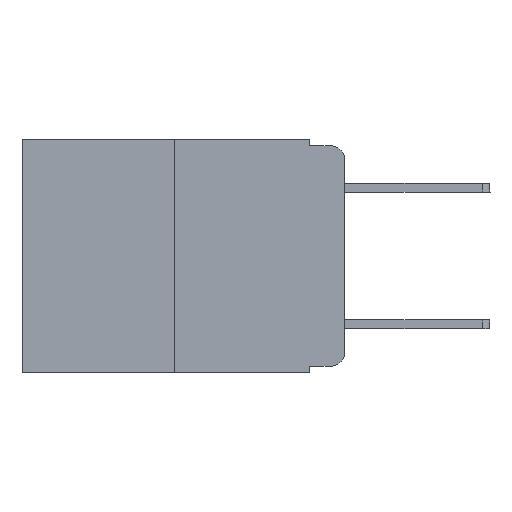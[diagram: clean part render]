
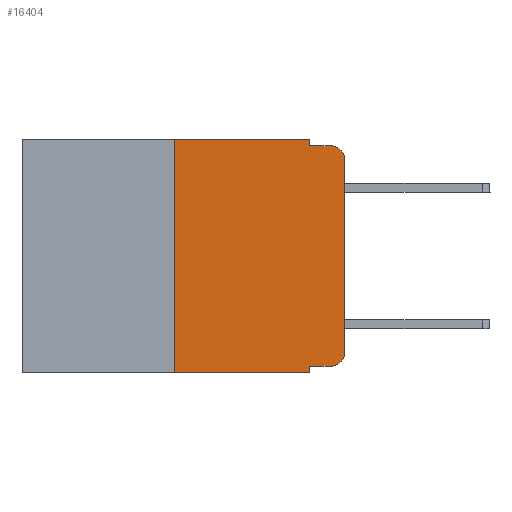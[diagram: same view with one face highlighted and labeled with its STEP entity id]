
A CAD part, left-side view. The second image highlights one B-rep face of the part: STEP entity #16404.
In plain terms, the highlighted planar face has unit normal (-1, 0, 0).
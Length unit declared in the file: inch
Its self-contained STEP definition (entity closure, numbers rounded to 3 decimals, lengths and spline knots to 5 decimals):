
#246 = AXIS2_PLACEMENT_3D ( 'NONE', #10239, #17850, #14669 ) ;
#283 = LINE ( 'NONE', #13062, #1094 ) ;
#313 = VERTEX_POINT ( 'NONE', #12540 ) ;
#344 = CARTESIAN_POINT ( 'NONE',  ( 0., 0.25, 0. ) ) ;
#580 = DIRECTION ( 'NONE',  ( 0., -1., 0. ) ) ;
#756 = VECTOR ( 'NONE', #9069, 39.37008 ) ;
#832 = ORIENTED_EDGE ( 'NONE', *, *, #17489, .T. ) ;
#1014 = CARTESIAN_POINT ( 'NONE',  ( 0., 0., -0.313 ) ) ;
#1094 = VECTOR ( 'NONE', #7331, 39.37008 ) ;
#1311 = ORIENTED_EDGE ( 'NONE', *, *, #4540, .T. ) ;
#1419 = DIRECTION ( 'NONE',  ( -1., 0., 0. ) ) ;
#1747 = CIRCLE ( 'NONE', #246, 0.02 ) ;
#2169 = EDGE_CURVE ( 'NONE', #313, #12812, #13133, .T. ) ;
#2287 = VECTOR ( 'NONE', #17711, 39.37008 ) ;
#2342 = EDGE_CURVE ( 'NONE', #17823, #13980, #2586, .T. ) ;
#2538 = DIRECTION ( 'NONE',  ( 0., 0., -1. ) ) ;
#2543 = DIRECTION ( 'NONE',  ( 0., -1., 0. ) ) ;
#2586 = LINE ( 'NONE', #13967, #7537 ) ;
#2757 = CARTESIAN_POINT ( 'NONE',  ( 0., 0.051, 0. ) ) ;
#2827 = CARTESIAN_POINT ( 'NONE',  ( 0., 0.02, -0.03 ) ) ;
#2892 = VERTEX_POINT ( 'NONE', #8205 ) ;
#3056 = VECTOR ( 'NONE', #3550, 39.37008 ) ;
#3317 = LINE ( 'NONE', #7725, #13115 ) ;
#3349 = LINE ( 'NONE', #17541, #756 ) ;
#3550 = DIRECTION ( 'NONE',  ( 0., -1., 0. ) ) ;
#4470 = EDGE_LOOP ( 'NONE', ( #15710, #832, #5228, #12486, #15642, #16694, #1311, #16005, #11245, #15691 ) ) ;
#4540 = EDGE_CURVE ( 'NONE', #14877, #2892, #9509, .T. ) ;
#5228 = ORIENTED_EDGE ( 'NONE', *, *, #2169, .F. ) ;
#5314 = DIRECTION ( 'NONE',  ( 0., 0., 1. ) ) ;
#5520 = CARTESIAN_POINT ( 'NONE',  ( 0., 0.473, 0. ) ) ;
#5703 = EDGE_CURVE ( 'NONE', #14877, #9881, #3349, .T. ) ;
#5923 = VERTEX_POINT ( 'NONE', #9895 ) ;
#6236 = CARTESIAN_POINT ( 'NONE',  ( 0., 0.051, 0. ) ) ;
#6400 = CARTESIAN_POINT ( 'NONE',  ( 0., 0.051, 0. ) ) ;
#6832 = CIRCLE ( 'NONE', #18574, 0.02 ) ;
#7331 = DIRECTION ( 'NONE',  ( 0., -1., 0. ) ) ;
#7537 = VECTOR ( 'NONE', #5314, 39.37008 ) ;
#7725 = CARTESIAN_POINT ( 'NONE',  ( 0., 0.051, -0.333 ) ) ;
#7865 = CARTESIAN_POINT ( 'NONE',  ( 0., 0., -0.03 ) ) ;
#8205 = CARTESIAN_POINT ( 'NONE',  ( 0., 0.051, -0.343 ) ) ;
#8352 = FACE_OUTER_BOUND ( 'NONE', #4470, .T. ) ;
#8901 = CARTESIAN_POINT ( 'NONE',  ( 0., 0.051, -0.01 ) ) ;
#9069 = DIRECTION ( 'NONE',  ( 0., 0., 1. ) ) ;
#9424 = CARTESIAN_POINT ( 'NONE',  ( 0., 0.051, -0.333 ) ) ;
#9485 = CARTESIAN_POINT ( 'NONE',  ( 0., 0.25, -0.343 ) ) ;
#9509 = LINE ( 'NONE', #18443, #13025 ) ;
#9881 = VERTEX_POINT ( 'NONE', #344 ) ;
#9895 = CARTESIAN_POINT ( 'NONE',  ( 0., 0.02, -0.333 ) ) ;
#10239 = CARTESIAN_POINT ( 'NONE',  ( 0., 0.02, -0.313 ) ) ;
#10451 = EDGE_CURVE ( 'NONE', #14421, #313, #17620, .T. ) ;
#11245 = ORIENTED_EDGE ( 'NONE', *, *, #12088, .T. ) ;
#11256 = DIRECTION ( 'NONE',  ( 1., 0., 0. ) ) ;
#11570 = VECTOR ( 'NONE', #14225, 39.37008 ) ;
#11762 = VERTEX_POINT ( 'NONE', #9424 ) ;
#12088 = EDGE_CURVE ( 'NONE', #11762, #5923, #3317, .T. ) ;
#12386 = EDGE_CURVE ( 'NONE', #9881, #14421, #283, .T. ) ;
#12486 = ORIENTED_EDGE ( 'NONE', *, *, #10451, .F. ) ;
#12540 = CARTESIAN_POINT ( 'NONE',  ( 0., 0.051, -0.01 ) ) ;
#12668 = PLANE ( 'NONE',  #13739 ) ;
#12812 = VERTEX_POINT ( 'NONE', #15974 ) ;
#13025 = VECTOR ( 'NONE', #2543, 39.37008 ) ;
#13062 = CARTESIAN_POINT ( 'NONE',  ( 0., 0.473, 0. ) ) ;
#13115 = VECTOR ( 'NONE', #580, 39.37008 ) ;
#13133 = LINE ( 'NONE', #8901, #3056 ) ;
#13739 = AXIS2_PLACEMENT_3D ( 'NONE', #5520, #11256, #17008 ) ;
#13967 = CARTESIAN_POINT ( 'NONE',  ( 0., 0., 0. ) ) ;
#13980 = VERTEX_POINT ( 'NONE', #7865 ) ;
#14220 = EDGE_CURVE ( 'NONE', #11762, #2892, #15635, .T. ) ;
#14225 = DIRECTION ( 'NONE',  ( 0., 0., -1. ) ) ;
#14421 = VERTEX_POINT ( 'NONE', #6400 ) ;
#14669 = DIRECTION ( 'NONE',  ( 0., 0., -1. ) ) ;
#14877 = VERTEX_POINT ( 'NONE', #9485 ) ;
#15635 = LINE ( 'NONE', #2757, #11570 ) ;
#15642 = ORIENTED_EDGE ( 'NONE', *, *, #12386, .F. ) ;
#15691 = ORIENTED_EDGE ( 'NONE', *, *, #17586, .T. ) ;
#15710 = ORIENTED_EDGE ( 'NONE', *, *, #2342, .T. ) ;
#15974 = CARTESIAN_POINT ( 'NONE',  ( 0., 0.02, -0.01 ) ) ;
#16005 = ORIENTED_EDGE ( 'NONE', *, *, #14220, .F. ) ;
#16404 = ADVANCED_FACE ( 'NONE', ( #8352 ), #12668, .F. ) ;
#16694 = ORIENTED_EDGE ( 'NONE', *, *, #5703, .F. ) ;
#17008 = DIRECTION ( 'NONE',  ( 0., 0., -1. ) ) ;
#17489 = EDGE_CURVE ( 'NONE', #13980, #12812, #6832, .T. ) ;
#17541 = CARTESIAN_POINT ( 'NONE',  ( 0., 0.25, 0. ) ) ;
#17586 = EDGE_CURVE ( 'NONE', #5923, #17823, #1747, .T. ) ;
#17620 = LINE ( 'NONE', #6236, #2287 ) ;
#17711 = DIRECTION ( 'NONE',  ( 0., 0., -1. ) ) ;
#17823 = VERTEX_POINT ( 'NONE', #1014 ) ;
#17850 = DIRECTION ( 'NONE',  ( -1., 0., 0. ) ) ;
#18443 = CARTESIAN_POINT ( 'NONE',  ( 0., 0.473, -0.343 ) ) ;
#18574 = AXIS2_PLACEMENT_3D ( 'NONE', #2827, #1419, #2538 ) ;
